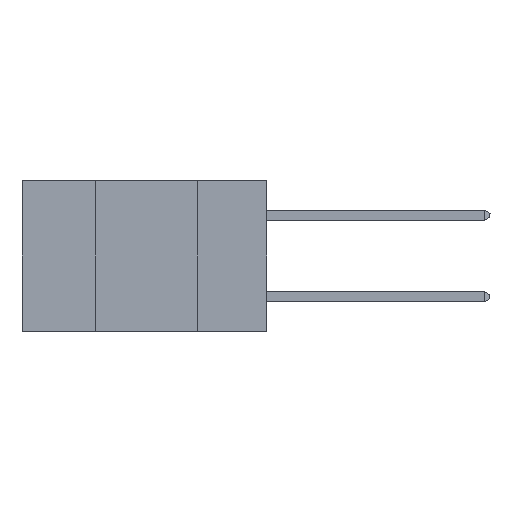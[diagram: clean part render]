
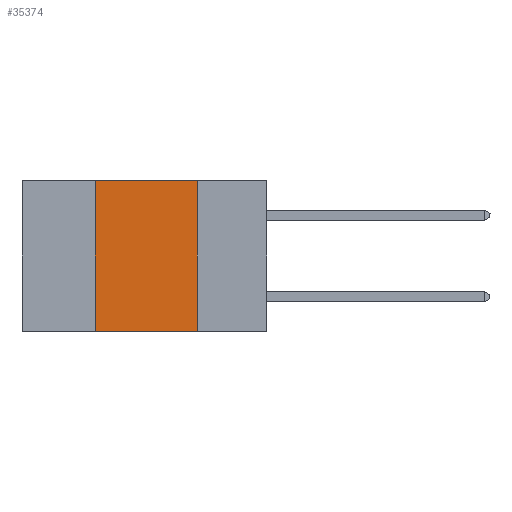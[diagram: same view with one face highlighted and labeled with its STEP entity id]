
A CAD part, left-side view. The second image highlights one B-rep face of the part: STEP entity #35374.
In plain terms, the highlighted planar face has unit normal (-1, 0, 0).
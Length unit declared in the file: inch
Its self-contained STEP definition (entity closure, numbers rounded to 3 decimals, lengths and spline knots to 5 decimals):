
#1063 = CARTESIAN_POINT ( 'NONE',  ( 0., 0.6, 0. ) ) ;
#1332 = CARTESIAN_POINT ( 'NONE',  ( 0., 0.42, 0. ) ) ;
#1585 = CARTESIAN_POINT ( 'NONE',  ( 0., 0.17, 0. ) ) ;
#1983 = CARTESIAN_POINT ( 'NONE',  ( 0., 0.6, -0.37 ) ) ;
#2131 = CARTESIAN_POINT ( 'NONE',  ( 0., 0.6, 0. ) ) ;
#3972 = DIRECTION ( 'NONE',  ( 1., 0., 0. ) ) ;
#4168 = FACE_OUTER_BOUND ( 'NONE', #24461, .T. ) ;
#4989 = ORIENTED_EDGE ( 'NONE', *, *, #31075, .T. ) ;
#5044 = CARTESIAN_POINT ( 'NONE',  ( 0., 0.17, -0.37 ) ) ;
#6633 = VERTEX_POINT ( 'NONE', #1332 ) ;
#6995 = ORIENTED_EDGE ( 'NONE', *, *, #37434, .F. ) ;
#10319 = VECTOR ( 'NONE', #34709, 39.37008 ) ;
#10886 = EDGE_CURVE ( 'NONE', #6633, #13269, #34869, .T. ) ;
#13269 = VERTEX_POINT ( 'NONE', #25765 ) ;
#14385 = CARTESIAN_POINT ( 'NONE',  ( 0., 0.42, 0. ) ) ;
#16067 = AXIS2_PLACEMENT_3D ( 'NONE', #1063, #3972, #36923 ) ;
#17001 = EDGE_CURVE ( 'NONE', #13269, #20915, #31976, .T. ) ;
#17099 = LINE ( 'NONE', #1983, #10319 ) ;
#18190 = VERTEX_POINT ( 'NONE', #37272 ) ;
#18720 = PLANE ( 'NONE',  #16067 ) ;
#20096 = ORIENTED_EDGE ( 'NONE', *, *, #17001, .F. ) ;
#20915 = VERTEX_POINT ( 'NONE', #5044 ) ;
#23216 = LINE ( 'NONE', #14385, #31844 ) ;
#24461 = EDGE_LOOP ( 'NONE', ( #20096, #33209, #6995, #4989 ) ) ;
#25679 = DIRECTION ( 'NONE',  ( 0., -1., 0. ) ) ;
#25765 = CARTESIAN_POINT ( 'NONE',  ( 0., 0.17, 0. ) ) ;
#25805 = VECTOR ( 'NONE', #26089, 39.37008 ) ;
#26089 = DIRECTION ( 'NONE',  ( 0., 0., -1. ) ) ;
#26350 = DIRECTION ( 'NONE',  ( 0., 0., 1. ) ) ;
#30375 = VECTOR ( 'NONE', #25679, 39.37008 ) ;
#31075 = EDGE_CURVE ( 'NONE', #18190, #20915, #17099, .T. ) ;
#31844 = VECTOR ( 'NONE', #26350, 39.37008 ) ;
#31976 = LINE ( 'NONE', #1585, #25805 ) ;
#33209 = ORIENTED_EDGE ( 'NONE', *, *, #10886, .F. ) ;
#34709 = DIRECTION ( 'NONE',  ( 0., -1., 0. ) ) ;
#34869 = LINE ( 'NONE', #2131, #30375 ) ;
#35374 = ADVANCED_FACE ( 'NONE', ( #4168 ), #18720, .F. ) ;
#36923 = DIRECTION ( 'NONE',  ( 0., 0., -1. ) ) ;
#37272 = CARTESIAN_POINT ( 'NONE',  ( 0., 0.42, -0.37 ) ) ;
#37434 = EDGE_CURVE ( 'NONE', #18190, #6633, #23216, .T. ) ;
